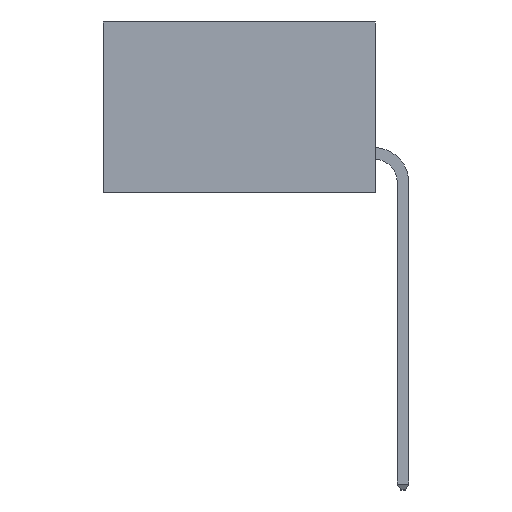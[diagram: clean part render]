
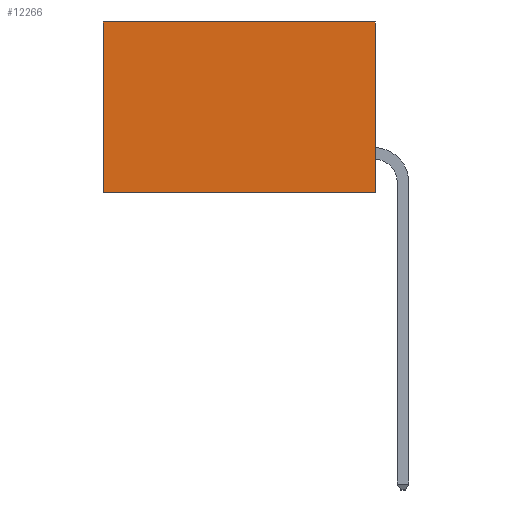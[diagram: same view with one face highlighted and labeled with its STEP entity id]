
A CAD part, left-side view. The second image highlights one B-rep face of the part: STEP entity #12266.
In plain terms, the highlighted planar face has unit normal (-1, 0, 0).
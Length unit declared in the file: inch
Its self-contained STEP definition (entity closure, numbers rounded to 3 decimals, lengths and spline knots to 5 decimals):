
#82 = VECTOR ( 'NONE', #9846, 39.37008 ) ;
#93 = LINE ( 'NONE', #1230, #9696 ) ;
#228 = DIRECTION ( 'NONE',  ( 0., 0., -1. ) ) ;
#357 = ORIENTED_EDGE ( 'NONE', *, *, #5189, .T. ) ;
#443 = CARTESIAN_POINT ( 'NONE',  ( 0.277, 0., -0.37 ) ) ;
#628 = EDGE_CURVE ( 'NONE', #10323, #11590, #8056, .T. ) ;
#675 = AXIS2_PLACEMENT_3D ( 'NONE', #5074, #6039, #228 ) ;
#1003 = CARTESIAN_POINT ( 'NONE',  ( 0.277, 0.59, 0. ) ) ;
#1228 = EDGE_CURVE ( 'NONE', #6483, #8589, #8480, .T. ) ;
#1230 = CARTESIAN_POINT ( 'NONE',  ( 0.277, 0., -0.37 ) ) ;
#1372 = DIRECTION ( 'NONE',  ( 0., 0., -1. ) ) ;
#2592 = CARTESIAN_POINT ( 'NONE',  ( 0.277, 0., 0. ) ) ;
#3601 = CARTESIAN_POINT ( 'NONE',  ( 0.277, 0., -0.37 ) ) ;
#4105 = CARTESIAN_POINT ( 'NONE',  ( 0.277, 0.59, -0.37 ) ) ;
#4714 = DIRECTION ( 'NONE',  ( 0., 0., -1. ) ) ;
#4763 = ORIENTED_EDGE ( 'NONE', *, *, #5194, .F. ) ;
#4794 = CARTESIAN_POINT ( 'NONE',  ( 0.277, 0.59, -0.37 ) ) ;
#4974 = VECTOR ( 'NONE', #4714, 39.37008 ) ;
#5064 = ORIENTED_EDGE ( 'NONE', *, *, #1228, .T. ) ;
#5074 = CARTESIAN_POINT ( 'NONE',  ( 0.277, 0., -0.37 ) ) ;
#5189 = EDGE_CURVE ( 'NONE', #8589, #11590, #5276, .T. ) ;
#5194 = EDGE_CURVE ( 'NONE', #6483, #10323, #93, .T. ) ;
#5276 = LINE ( 'NONE', #4794, #4974 ) ;
#6009 = VECTOR ( 'NONE', #10104, 39.37008 ) ;
#6039 = DIRECTION ( 'NONE',  ( 1., 0., 0. ) ) ;
#6411 = FACE_OUTER_BOUND ( 'NONE', #8994, .T. ) ;
#6483 = VERTEX_POINT ( 'NONE', #9094 ) ;
#8056 = LINE ( 'NONE', #443, #82 ) ;
#8480 = LINE ( 'NONE', #2592, #6009 ) ;
#8589 = VERTEX_POINT ( 'NONE', #1003 ) ;
#8994 = EDGE_LOOP ( 'NONE', ( #357, #10501, #4763, #5064 ) ) ;
#9094 = CARTESIAN_POINT ( 'NONE',  ( 0.277, 0., 0. ) ) ;
#9696 = VECTOR ( 'NONE', #1372, 39.37008 ) ;
#9846 = DIRECTION ( 'NONE',  ( 0., 1., 0. ) ) ;
#10104 = DIRECTION ( 'NONE',  ( 0., 1., 0. ) ) ;
#10323 = VERTEX_POINT ( 'NONE', #3601 ) ;
#10501 = ORIENTED_EDGE ( 'NONE', *, *, #628, .F. ) ;
#10718 = PLANE ( 'NONE',  #675 ) ;
#11590 = VERTEX_POINT ( 'NONE', #4105 ) ;
#12266 = ADVANCED_FACE ( 'NONE', ( #6411 ), #10718, .F. ) ;
